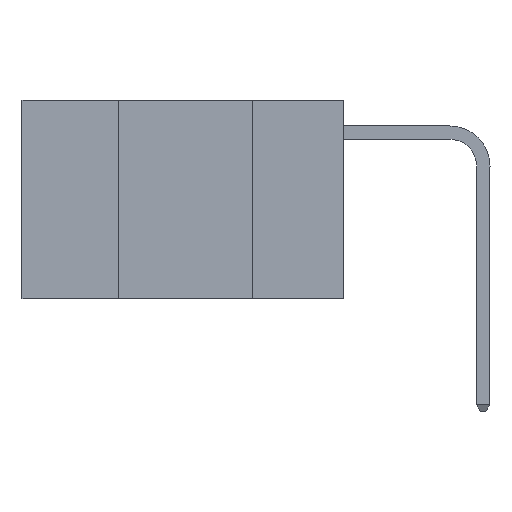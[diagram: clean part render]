
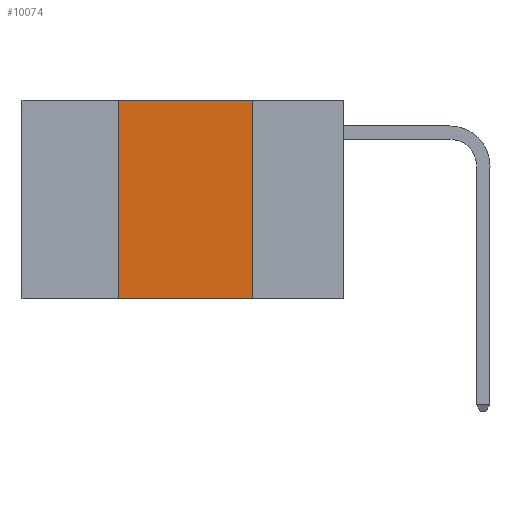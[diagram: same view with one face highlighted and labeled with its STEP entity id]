
A CAD part, left-side view. The second image highlights one B-rep face of the part: STEP entity #10074.
In plain terms, the highlighted planar face has unit normal (-1, 0, 0).
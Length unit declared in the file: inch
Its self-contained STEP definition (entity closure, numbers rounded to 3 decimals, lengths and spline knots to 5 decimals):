
#38 = DIRECTION ( 'NONE',  ( 0., -1., 0. ) ) ;
#65 = CARTESIAN_POINT ( 'NONE',  ( 0., 0.6, 0. ) ) ;
#311 = VECTOR ( 'NONE', #38, 39.37008 ) ;
#958 = ORIENTED_EDGE ( 'NONE', *, *, #17319, .F. ) ;
#1086 = EDGE_LOOP ( 'NONE', ( #5281, #958, #7396, #12409 ) ) ;
#1193 = EDGE_CURVE ( 'NONE', #4158, #11224, #14957, .T. ) ;
#3410 = CARTESIAN_POINT ( 'NONE',  ( 0., 0.42, 0. ) ) ;
#4022 = CARTESIAN_POINT ( 'NONE',  ( 0., 0.42, 0. ) ) ;
#4158 = VERTEX_POINT ( 'NONE', #17635 ) ;
#4967 = VERTEX_POINT ( 'NONE', #16299 ) ;
#5281 = ORIENTED_EDGE ( 'NONE', *, *, #7032, .F. ) ;
#5781 = VECTOR ( 'NONE', #9269, 39.37008 ) ;
#6768 = EDGE_CURVE ( 'NONE', #4158, #4967, #14641, .T. ) ;
#7032 = EDGE_CURVE ( 'NONE', #10096, #4967, #21984, .T. ) ;
#7294 = PLANE ( 'NONE',  #11953 ) ;
#7396 = ORIENTED_EDGE ( 'NONE', *, *, #1193, .F. ) ;
#7429 = CARTESIAN_POINT ( 'NONE',  ( 0., 0.6, -0.37 ) ) ;
#8263 = DIRECTION ( 'NONE',  ( 0., 0., -1. ) ) ;
#9074 = DIRECTION ( 'NONE',  ( 0., 0., -1. ) ) ;
#9269 = DIRECTION ( 'NONE',  ( 0., -1., 0. ) ) ;
#10074 = ADVANCED_FACE ( 'NONE', ( #13981 ), #7294, .F. ) ;
#10096 = VERTEX_POINT ( 'NONE', #21314 ) ;
#10282 = VECTOR ( 'NONE', #14690, 39.37008 ) ;
#11224 = VERTEX_POINT ( 'NONE', #3410 ) ;
#11953 = AXIS2_PLACEMENT_3D ( 'NONE', #65, #19559, #9074 ) ;
#12409 = ORIENTED_EDGE ( 'NONE', *, *, #6768, .T. ) ;
#13981 = FACE_OUTER_BOUND ( 'NONE', #1086, .T. ) ;
#14289 = CARTESIAN_POINT ( 'NONE',  ( 0., 0.6, 0. ) ) ;
#14641 = LINE ( 'NONE', #7429, #5781 ) ;
#14690 = DIRECTION ( 'NONE',  ( 0., 0., 1. ) ) ;
#14957 = LINE ( 'NONE', #4022, #10282 ) ;
#16299 = CARTESIAN_POINT ( 'NONE',  ( 0., 0.17, -0.37 ) ) ;
#17319 = EDGE_CURVE ( 'NONE', #11224, #10096, #19160, .T. ) ;
#17635 = CARTESIAN_POINT ( 'NONE',  ( 0., 0.42, -0.37 ) ) ;
#18749 = CARTESIAN_POINT ( 'NONE',  ( 0., 0.17, 0. ) ) ;
#18978 = VECTOR ( 'NONE', #8263, 39.37008 ) ;
#19160 = LINE ( 'NONE', #14289, #311 ) ;
#19559 = DIRECTION ( 'NONE',  ( 1., 0., 0. ) ) ;
#21314 = CARTESIAN_POINT ( 'NONE',  ( 0., 0.17, 0. ) ) ;
#21984 = LINE ( 'NONE', #18749, #18978 ) ;
